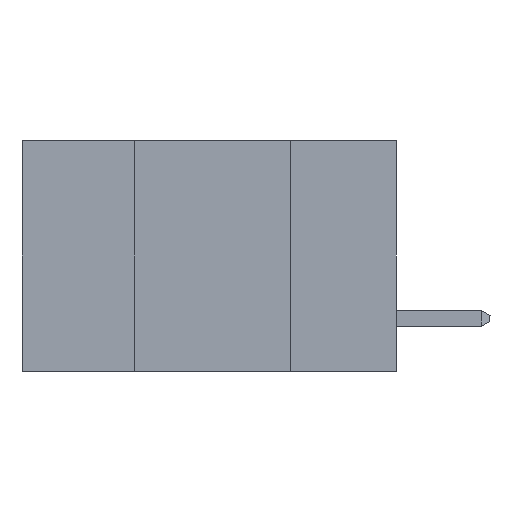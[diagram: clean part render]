
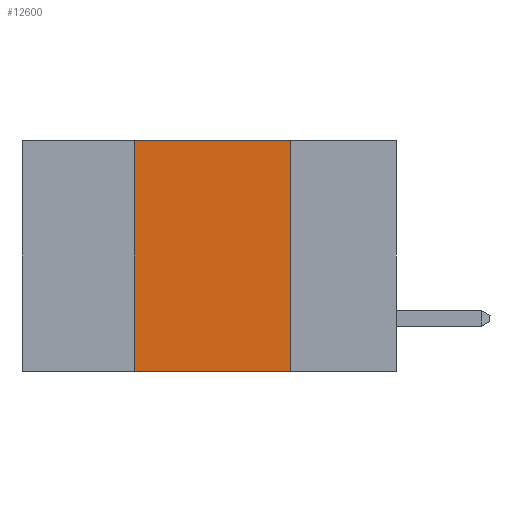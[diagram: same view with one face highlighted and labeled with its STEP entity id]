
A CAD part, left-side view. The second image highlights one B-rep face of the part: STEP entity #12600.
In plain terms, the highlighted planar face has unit normal (-1, 0, 0).
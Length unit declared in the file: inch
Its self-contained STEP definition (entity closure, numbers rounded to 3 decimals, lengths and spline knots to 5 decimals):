
#1196 = DIRECTION ( 'NONE',  ( 0., -1., 0. ) ) ;
#1281 = LINE ( 'NONE', #6868, #17148 ) ;
#3278 = VERTEX_POINT ( 'NONE', #17814 ) ;
#3334 = CARTESIAN_POINT ( 'NONE',  ( 0., 0.6, 0. ) ) ;
#3684 = VECTOR ( 'NONE', #8337, 39.37008 ) ;
#5858 = LINE ( 'NONE', #9903, #3684 ) ;
#6090 = PLANE ( 'NONE',  #12361 ) ;
#6868 = CARTESIAN_POINT ( 'NONE',  ( 0., 0.6, -0.37 ) ) ;
#6996 = EDGE_CURVE ( 'NONE', #16141, #13125, #11358, .T. ) ;
#7486 = ORIENTED_EDGE ( 'NONE', *, *, #17359, .F. ) ;
#8337 = DIRECTION ( 'NONE',  ( 0., 0., -1. ) ) ;
#9859 = VECTOR ( 'NONE', #9984, 39.37008 ) ;
#9903 = CARTESIAN_POINT ( 'NONE',  ( 0., 0.17, -0.37 ) ) ;
#9984 = DIRECTION ( 'NONE',  ( 0., 0., 1. ) ) ;
#10165 = CARTESIAN_POINT ( 'NONE',  ( 0., 0.42, -0.37 ) ) ;
#10428 = ORIENTED_EDGE ( 'NONE', *, *, #6996, .F. ) ;
#11008 = VECTOR ( 'NONE', #14034, 39.37008 ) ;
#11358 = LINE ( 'NONE', #10165, #9859 ) ;
#11373 = VERTEX_POINT ( 'NONE', #15998 ) ;
#12283 = ORIENTED_EDGE ( 'NONE', *, *, #17183, .T. ) ;
#12361 = AXIS2_PLACEMENT_3D ( 'NONE', #3334, #17472, #14541 ) ;
#12600 = ADVANCED_FACE ( 'NONE', ( #13243 ), #6090, .F. ) ;
#12923 = LINE ( 'NONE', #16701, #11008 ) ;
#13125 = VERTEX_POINT ( 'NONE', #13657 ) ;
#13243 = FACE_OUTER_BOUND ( 'NONE', #14962, .T. ) ;
#13657 = CARTESIAN_POINT ( 'NONE',  ( 0., 0.42, 0. ) ) ;
#14034 = DIRECTION ( 'NONE',  ( 0., -1., 0. ) ) ;
#14503 = CARTESIAN_POINT ( 'NONE',  ( 0., 0.42, -0.37 ) ) ;
#14541 = DIRECTION ( 'NONE',  ( 0., 0., -1. ) ) ;
#14962 = EDGE_LOOP ( 'NONE', ( #7486, #16037, #10428, #12283 ) ) ;
#15998 = CARTESIAN_POINT ( 'NONE',  ( 0., 0.17, 0. ) ) ;
#16037 = ORIENTED_EDGE ( 'NONE', *, *, #17395, .F. ) ;
#16141 = VERTEX_POINT ( 'NONE', #14503 ) ;
#16701 = CARTESIAN_POINT ( 'NONE',  ( 0., 0.6, 0. ) ) ;
#17148 = VECTOR ( 'NONE', #1196, 39.37008 ) ;
#17183 = EDGE_CURVE ( 'NONE', #16141, #3278, #1281, .T. ) ;
#17359 = EDGE_CURVE ( 'NONE', #11373, #3278, #5858, .T. ) ;
#17395 = EDGE_CURVE ( 'NONE', #13125, #11373, #12923, .T. ) ;
#17472 = DIRECTION ( 'NONE',  ( 1., 0., 0. ) ) ;
#17814 = CARTESIAN_POINT ( 'NONE',  ( 0., 0.17, -0.37 ) ) ;
